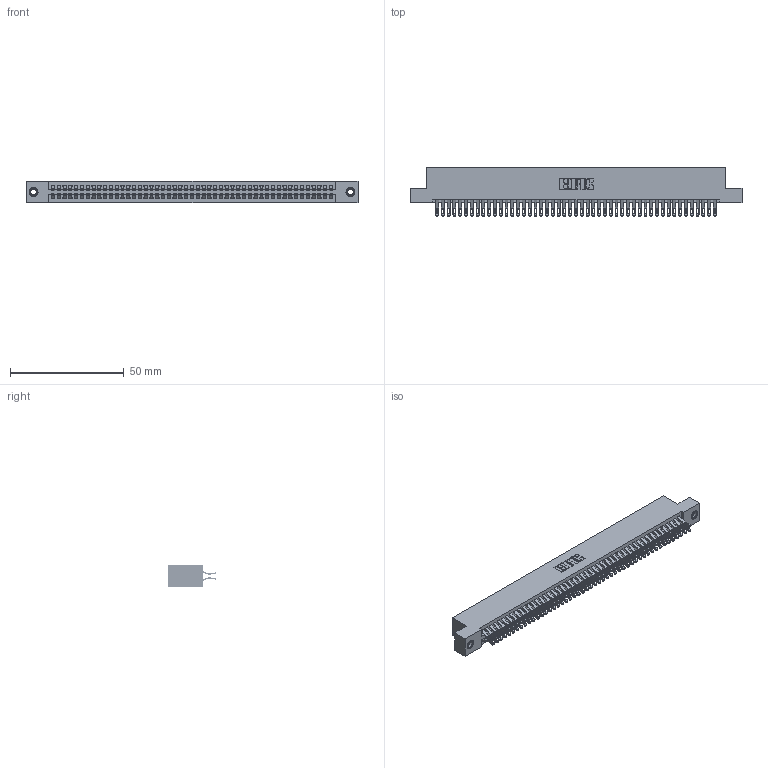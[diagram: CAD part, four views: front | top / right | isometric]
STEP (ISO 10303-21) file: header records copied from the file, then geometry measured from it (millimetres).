
FILE_DESCRIPTION (( 'STEP AP203' ), '1' );
FILE_NAME ('345-098-555-207.STEP', '2019-11-02T12:21:57', ( '' ), ( '' ), 'SwSTEP 2.0', 'SolidWorks 2016', '' );
FILE_SCHEMA (( 'CONFIG_CONTROL_DESIGN' ));
Length unit declared in the file: inch
Products named in the file (4): 345-250-001_345-250-005-103; 345-292-001_555 Tail; 345 Part_Flush Mounting Lugs - 0.156 Dia-TI; 345-098-555-207
Assembly tree (101 placements, depth 2):
  345-098-555-207
    345 Part_Flush Mounting Lugs - 0.156 Dia-TI
    345-292-001_555 Tail  x98
    345-250-001_345-250-005-103  x2
Bounding box: 145.67 x 21.13 x 9.4 mm (x, y, z)
Volume: 14486.1 mm3; surface area: 22565.1 mm2
Topology: 101 solids, 101 shells, 5674 faces, 17823 edges, 11874 vertices
Faces by surface type: plane 3150, cylinder 2508, cone 12, torus 4
Entity records: 39016 total; most frequent: CARTESIAN_POINT 6549, ORIENTED_EDGE 6446, DIRECTION 5761, EDGE_CURVE 3223, VECTOR 2855, LINE 2855, VERTEX_POINT 2144, AXIS2_PLACEMENT_3D 1453
